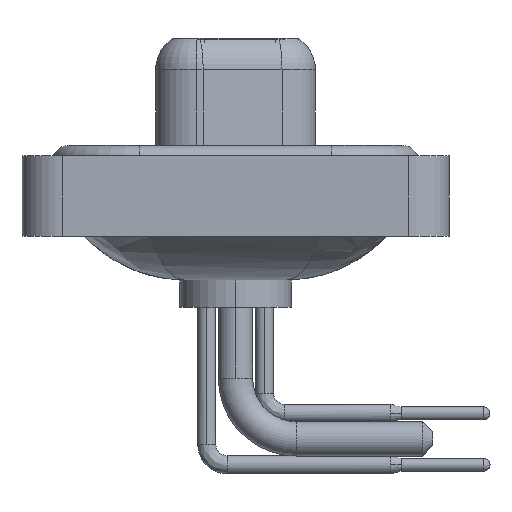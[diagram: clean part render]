
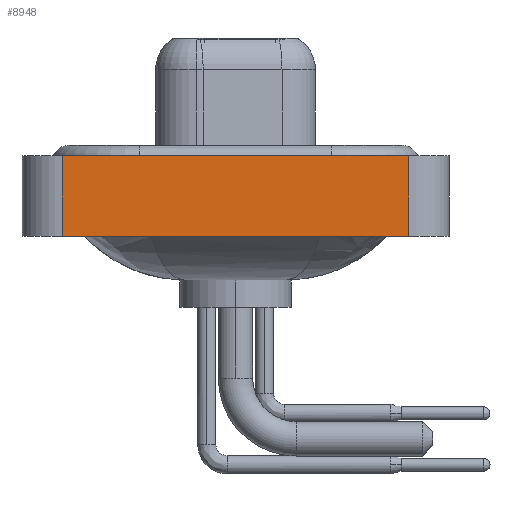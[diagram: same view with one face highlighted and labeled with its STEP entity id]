
A CAD part, left-side view. The second image highlights one B-rep face of the part: STEP entity #8948.
In plain terms, the highlighted planar face has unit normal (-1, 0, 0).
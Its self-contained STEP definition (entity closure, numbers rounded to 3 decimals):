
#130 = CARTESIAN_POINT ( 'NONE',  ( -7.35, -8.55, -3.6 ) ) ;
#463 = EDGE_CURVE ( 'NONE', #11428, #15476, #5580, .T. ) ;
#575 = VERTEX_POINT ( 'NONE', #6314 ) ;
#2283 = CARTESIAN_POINT ( 'NONE',  ( -7.35, -8.55, -3.6 ) ) ;
#2723 = FACE_OUTER_BOUND ( 'NONE', #9182, .T. ) ;
#2821 = PLANE ( 'NONE',  #14409 ) ;
#3698 = ORIENTED_EDGE ( 'NONE', *, *, #16500, .F. ) ;
#3762 = CARTESIAN_POINT ( 'NONE',  ( -7.35, -8.55, 0.4 ) ) ;
#3998 = DIRECTION ( 'NONE',  ( 0., -1., 0. ) ) ;
#4037 = CARTESIAN_POINT ( 'NONE',  ( -7.35, 8.55, -3.6 ) ) ;
#5093 = LINE ( 'NONE', #130, #19338 ) ;
#5580 = LINE ( 'NONE', #12031, #13707 ) ;
#5842 = LINE ( 'NONE', #4037, #13262 ) ;
#5891 = EDGE_CURVE ( 'NONE', #15476, #12301, #5093, .T. ) ;
#6314 = CARTESIAN_POINT ( 'NONE',  ( -7.35, 8.55, 0.4 ) ) ;
#6329 = ORIENTED_EDGE ( 'NONE', *, *, #463, .T. ) ;
#7641 = VECTOR ( 'NONE', #10321, 1000. ) ;
#8715 = EDGE_CURVE ( 'NONE', #575, #12301, #16997, .T. ) ;
#8948 = ADVANCED_FACE ( 'NONE', ( #2723 ), #2821, .T. ) ;
#9151 = CARTESIAN_POINT ( 'NONE',  ( -7.35, -8.55, -3.6 ) ) ;
#9182 = EDGE_LOOP ( 'NONE', ( #19059, #18961, #3698, #6329 ) ) ;
#10321 = DIRECTION ( 'NONE',  ( 0., -1., 0. ) ) ;
#11428 = VERTEX_POINT ( 'NONE', #14831 ) ;
#12031 = CARTESIAN_POINT ( 'NONE',  ( -7.35, -8.55, -3.6 ) ) ;
#12301 = VERTEX_POINT ( 'NONE', #3762 ) ;
#13262 = VECTOR ( 'NONE', #15573, 1000. ) ;
#13707 = VECTOR ( 'NONE', #3998, 1000. ) ;
#14409 = AXIS2_PLACEMENT_3D ( 'NONE', #9151, #15625, #17323 ) ;
#14831 = CARTESIAN_POINT ( 'NONE',  ( -7.35, 8.55, -3.6 ) ) ;
#15476 = VERTEX_POINT ( 'NONE', #2283 ) ;
#15573 = DIRECTION ( 'NONE',  ( 0., 0., 1. ) ) ;
#15625 = DIRECTION ( 'NONE',  ( -1., 0., 0. ) ) ;
#16500 = EDGE_CURVE ( 'NONE', #11428, #575, #5842, .T. ) ;
#16997 = LINE ( 'NONE', #19876, #7641 ) ;
#17323 = DIRECTION ( 'NONE',  ( 0., 0., 1. ) ) ;
#18105 = DIRECTION ( 'NONE',  ( 0., 0., 1. ) ) ;
#18961 = ORIENTED_EDGE ( 'NONE', *, *, #8715, .F. ) ;
#19059 = ORIENTED_EDGE ( 'NONE', *, *, #5891, .T. ) ;
#19338 = VECTOR ( 'NONE', #18105, 1000. ) ;
#19876 = CARTESIAN_POINT ( 'NONE',  ( -7.35, -8.55, 0.4 ) ) ;
